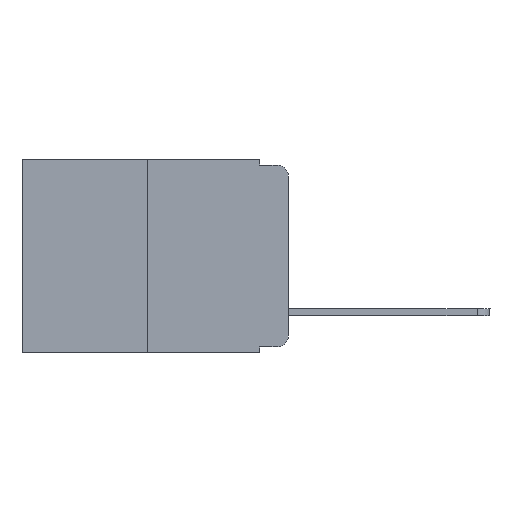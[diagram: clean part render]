
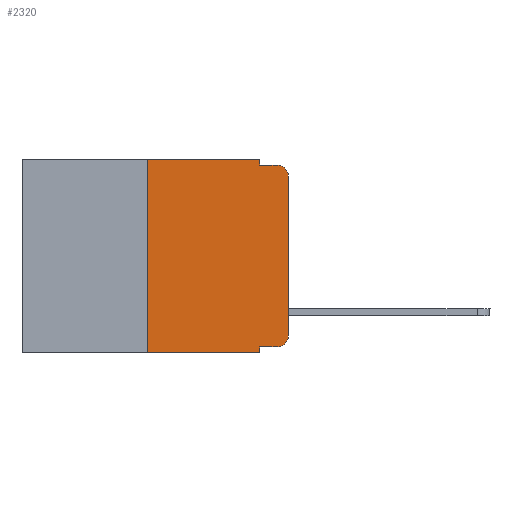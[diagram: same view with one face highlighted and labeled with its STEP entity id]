
A CAD part, left-side view. The second image highlights one B-rep face of the part: STEP entity #2320.
In plain terms, the highlighted planar face has unit normal (-1, 0, 0).
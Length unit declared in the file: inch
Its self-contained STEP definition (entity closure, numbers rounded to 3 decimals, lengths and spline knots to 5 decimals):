
#17 = VERTEX_POINT ( 'NONE', #1152 ) ;
#96 = ORIENTED_EDGE ( 'NONE', *, *, #309, .T. ) ;
#168 = EDGE_CURVE ( 'NONE', #7916, #4947, #10702, .T. ) ;
#309 = EDGE_CURVE ( 'NONE', #8756, #7324, #8365, .T. ) ;
#321 = LINE ( 'NONE', #4617, #5415 ) ;
#379 = DIRECTION ( 'NONE',  ( 0., 0., -1. ) ) ;
#447 = EDGE_CURVE ( 'NONE', #8716, #10665, #321, .T. ) ;
#495 = CARTESIAN_POINT ( 'NONE',  ( 0., 0.051, -0.01 ) ) ;
#557 = ORIENTED_EDGE ( 'NONE', *, *, #3480, .T. ) ;
#582 = CARTESIAN_POINT ( 'NONE',  ( 0., 0.051, -0.01 ) ) ;
#700 = DIRECTION ( 'NONE',  ( 1., 0., 0. ) ) ;
#824 = CARTESIAN_POINT ( 'NONE',  ( 0., 0.051, -0.343 ) ) ;
#873 = VECTOR ( 'NONE', #5333, 39.37008 ) ;
#957 = ORIENTED_EDGE ( 'NONE', *, *, #3903, .F. ) ;
#1152 = CARTESIAN_POINT ( 'NONE',  ( 0., 0.02, -0.01 ) ) ;
#1353 = DIRECTION ( 'NONE',  ( 0., -1., 0. ) ) ;
#1399 = EDGE_CURVE ( 'NONE', #8716, #9999, #10597, .T. ) ;
#1530 = CARTESIAN_POINT ( 'NONE',  ( 0., 0.051, -0.333 ) ) ;
#1557 = AXIS2_PLACEMENT_3D ( 'NONE', #3760, #5454, #7785 ) ;
#1621 = CARTESIAN_POINT ( 'NONE',  ( 0., 0.25, -0.343 ) ) ;
#1783 = ORIENTED_EDGE ( 'NONE', *, *, #1399, .T. ) ;
#2112 = AXIS2_PLACEMENT_3D ( 'NONE', #5485, #4722, #10473 ) ;
#2266 = VECTOR ( 'NONE', #1353, 39.37008 ) ;
#2320 = ADVANCED_FACE ( 'NONE', ( #7064 ), #10375, .F. ) ;
#2621 = ORIENTED_EDGE ( 'NONE', *, *, #447, .F. ) ;
#2715 = VECTOR ( 'NONE', #9057, 39.37008 ) ;
#3004 = VECTOR ( 'NONE', #8095, 39.37008 ) ;
#3143 = DIRECTION ( 'NONE',  ( 0., 0., -1. ) ) ;
#3394 = ORIENTED_EDGE ( 'NONE', *, *, #9651, .T. ) ;
#3480 = EDGE_CURVE ( 'NONE', #5354, #10665, #6739, .T. ) ;
#3760 = CARTESIAN_POINT ( 'NONE',  ( 0., 0.02, -0.03 ) ) ;
#3885 = ORIENTED_EDGE ( 'NONE', *, *, #9268, .F. ) ;
#3903 = EDGE_CURVE ( 'NONE', #6496, #17, #4719, .T. ) ;
#4065 = CARTESIAN_POINT ( 'NONE',  ( 0., 0.051, 0. ) ) ;
#4462 = VECTOR ( 'NONE', #10490, 39.37008 ) ;
#4543 = CARTESIAN_POINT ( 'NONE',  ( 0., 0.25, 0. ) ) ;
#4617 = CARTESIAN_POINT ( 'NONE',  ( 0., 0.051, 0. ) ) ;
#4689 = CIRCLE ( 'NONE', #1557, 0.02 ) ;
#4719 = LINE ( 'NONE', #582, #2266 ) ;
#4722 = DIRECTION ( 'NONE',  ( -1., 0., 0. ) ) ;
#4771 = AXIS2_PLACEMENT_3D ( 'NONE', #7935, #700, #3143 ) ;
#4837 = CARTESIAN_POINT ( 'NONE',  ( 0., 0.25, 0. ) ) ;
#4936 = CARTESIAN_POINT ( 'NONE',  ( 0., 0.051, 0. ) ) ;
#4947 = VERTEX_POINT ( 'NONE', #4065 ) ;
#5145 = CARTESIAN_POINT ( 'NONE',  ( 0., 0.051, -0.333 ) ) ;
#5155 = EDGE_CURVE ( 'NONE', #9999, #8756, #6785, .T. ) ;
#5333 = DIRECTION ( 'NONE',  ( 0., -1., 0. ) ) ;
#5354 = VERTEX_POINT ( 'NONE', #1621 ) ;
#5415 = VECTOR ( 'NONE', #379, 39.37008 ) ;
#5454 = DIRECTION ( 'NONE',  ( -1., 0., 0. ) ) ;
#5485 = CARTESIAN_POINT ( 'NONE',  ( 0., 0.02, -0.313 ) ) ;
#6217 = ORIENTED_EDGE ( 'NONE', *, *, #6631, .F. ) ;
#6242 = VECTOR ( 'NONE', #7959, 39.37008 ) ;
#6252 = CARTESIAN_POINT ( 'NONE',  ( 0., 0.473, -0.343 ) ) ;
#6496 = VERTEX_POINT ( 'NONE', #495 ) ;
#6631 = EDGE_CURVE ( 'NONE', #4947, #6496, #9872, .T. ) ;
#6739 = LINE ( 'NONE', #6252, #873 ) ;
#6775 = CARTESIAN_POINT ( 'NONE',  ( 0., 0., -0.313 ) ) ;
#6785 = CIRCLE ( 'NONE', #2112, 0.02 ) ;
#6801 = ORIENTED_EDGE ( 'NONE', *, *, #5155, .T. ) ;
#7064 = FACE_OUTER_BOUND ( 'NONE', #7472, .T. ) ;
#7324 = VERTEX_POINT ( 'NONE', #9317 ) ;
#7472 = EDGE_LOOP ( 'NONE', ( #96, #3394, #957, #6217, #7527, #3885, #557, #2621, #1783, #6801 ) ) ;
#7527 = ORIENTED_EDGE ( 'NONE', *, *, #168, .F. ) ;
#7785 = DIRECTION ( 'NONE',  ( 0., 0., -1. ) ) ;
#7916 = VERTEX_POINT ( 'NONE', #4837 ) ;
#7935 = CARTESIAN_POINT ( 'NONE',  ( 0., 0.473, 0. ) ) ;
#7959 = DIRECTION ( 'NONE',  ( 0., 0., 1. ) ) ;
#8095 = DIRECTION ( 'NONE',  ( 0., -1., 0. ) ) ;
#8365 = LINE ( 'NONE', #8466, #9238 ) ;
#8466 = CARTESIAN_POINT ( 'NONE',  ( 0., 0., 0. ) ) ;
#8716 = VERTEX_POINT ( 'NONE', #5145 ) ;
#8727 = CARTESIAN_POINT ( 'NONE',  ( 0., 0.02, -0.333 ) ) ;
#8756 = VERTEX_POINT ( 'NONE', #6775 ) ;
#9004 = CARTESIAN_POINT ( 'NONE',  ( 0., 0.473, 0. ) ) ;
#9057 = DIRECTION ( 'NONE',  ( 0., 0., -1. ) ) ;
#9238 = VECTOR ( 'NONE', #9984, 39.37008 ) ;
#9268 = EDGE_CURVE ( 'NONE', #5354, #7916, #10557, .T. ) ;
#9317 = CARTESIAN_POINT ( 'NONE',  ( 0., 0., -0.03 ) ) ;
#9651 = EDGE_CURVE ( 'NONE', #7324, #17, #4689, .T. ) ;
#9872 = LINE ( 'NONE', #4936, #2715 ) ;
#9984 = DIRECTION ( 'NONE',  ( 0., 0., 1. ) ) ;
#9999 = VERTEX_POINT ( 'NONE', #8727 ) ;
#10375 = PLANE ( 'NONE',  #4771 ) ;
#10473 = DIRECTION ( 'NONE',  ( 0., 0., -1. ) ) ;
#10490 = DIRECTION ( 'NONE',  ( 0., -1., 0. ) ) ;
#10557 = LINE ( 'NONE', #4543, #6242 ) ;
#10597 = LINE ( 'NONE', #1530, #4462 ) ;
#10665 = VERTEX_POINT ( 'NONE', #824 ) ;
#10702 = LINE ( 'NONE', #9004, #3004 ) ;
